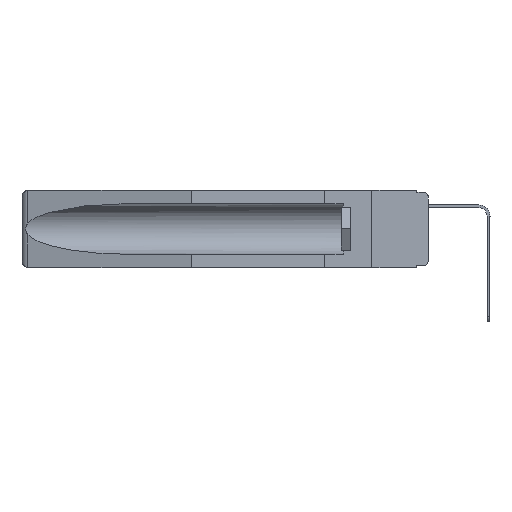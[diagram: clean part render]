
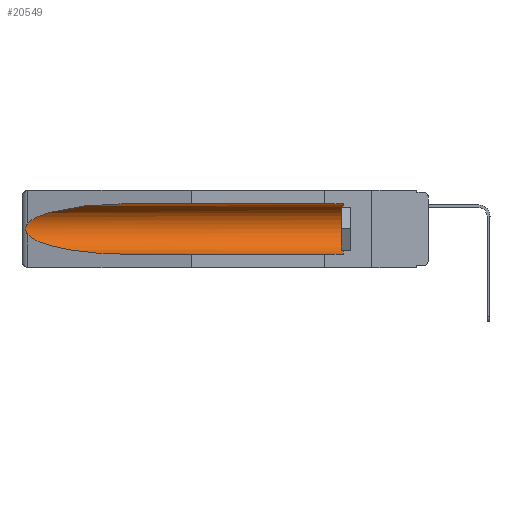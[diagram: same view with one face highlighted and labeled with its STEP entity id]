
A CAD part, left-side view. The second image highlights one B-rep face of the part: STEP entity #20549.
In plain terms, the highlighted cylindrical face has radius 2.857 mm (diameter 5.715 mm), a partial arc.
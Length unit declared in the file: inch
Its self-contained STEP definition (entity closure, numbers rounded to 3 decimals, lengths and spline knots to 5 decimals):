
#26 = VERTEX_POINT ( 'NONE', #24285 ) ;
#1350 = VERTEX_POINT ( 'NONE', #5769 ) ;
#1535 = CARTESIAN_POINT ( 'NONE',  ( 0.155, 1.07973, -0.284 ) ) ;
#2356 = ORIENTED_EDGE ( 'NONE', *, *, #2501, .T. ) ;
#2501 = EDGE_CURVE ( 'NONE', #20024, #16948, #13579, .T. ) ;
#2615 = CARTESIAN_POINT ( 'NONE',  ( 0.26654, 1.53092, -0.15636 ) ) ;
#2999 = FACE_OUTER_BOUND ( 'NONE', #20802, .T. ) ;
#3125 = CARTESIAN_POINT ( 'NONE',  ( 0.2675, 1.53308, -0.17534 ) ) ;
#3566 = ORIENTED_EDGE ( 'NONE', *, *, #14625, .T. ) ;
#3877 = CARTESIAN_POINT ( 'NONE',  ( 0.155, -0.30754, -0.284 ) ) ;
#4332 = CARTESIAN_POINT ( 'NONE',  ( 0.155, -0.30754, -0.1715 ) ) ;
#4775 = CARTESIAN_POINT ( 'NONE',  ( 0.26537, 1.52718, -0.19328 ) ) ;
#5769 = CARTESIAN_POINT ( 'NONE',  ( 0.155, 0.126, -0.284 ) ) ;
#6093 = ORIENTED_EDGE ( 'NONE', *, *, #7847, .F. ) ;
#6315 = CARTESIAN_POINT ( 'NONE',  ( 0.155, -0.30754, -0.059 ) ) ;
#6338 = DIRECTION ( 'NONE',  ( 0., 1., 0. ) ) ;
#6850 =( BOUNDED_CURVE ( )  B_SPLINE_CURVE ( 3, ( #9888, #23313, #19418, #12179 ),
 .UNSPECIFIED., .F., .F. ) 
 B_SPLINE_CURVE_WITH_KNOTS ( ( 4, 4 ),
 ( 4.71239, 6.08839 ),
 .UNSPECIFIED. ) 
 CURVE ( )  GEOMETRIC_REPRESENTATION_ITEM ( )  RATIONAL_B_SPLINE_CURVE ( ( 1., 0.848, 0.848, 1. ) ) 
 REPRESENTATION_ITEM ( '' )  );
#6964 = CARTESIAN_POINT ( 'NONE',  ( 0.26655, 1.53094, -0.18657 ) ) ;
#7096 = CARTESIAN_POINT ( 'NONE',  ( 0.21114, 1.30732, -0.284 ) ) ;
#7478 = CYLINDRICAL_SURFACE ( 'NONE', #15297, 0.1125 ) ;
#7492 = DIRECTION ( 'NONE',  ( 0., -1., 0. ) ) ;
#7847 = EDGE_CURVE ( 'NONE', #1350, #23881, #13868, .T. ) ;
#8426 = CARTESIAN_POINT ( 'NONE',  ( 0.26537, 1.52718, -0.14972 ) ) ;
#8512 = CARTESIAN_POINT ( 'NONE',  ( 0.2673, 1.5327, -0.16383 ) ) ;
#8907 = CARTESIAN_POINT ( 'NONE',  ( 0.155, 1.07973, -0.284 ) ) ;
#9697 = AXIS2_PLACEMENT_3D ( 'NONE', #18843, #7492, #20726 ) ;
#9840 = EDGE_CURVE ( 'NONE', #1350, #20024, #19397, .T. ) ;
#9888 = CARTESIAN_POINT ( 'NONE',  ( 0.155, 1.07973, -0.059 ) ) ;
#10599 = CARTESIAN_POINT ( 'NONE',  ( 0.2673, 1.53269, -0.17917 ) ) ;
#11161 = CARTESIAN_POINT ( 'NONE',  ( 0.26537, 1.52718, -0.14972 ) ) ;
#11179 = VECTOR ( 'NONE', #17166, 39.37008 ) ;
#12013 = EDGE_CURVE ( 'NONE', #16948, #20307, #6850, .T. ) ;
#12179 = CARTESIAN_POINT ( 'NONE',  ( 0.26537, 1.52718, -0.14972 ) ) ;
#12754 = CARTESIAN_POINT ( 'NONE',  ( 0.2675, 1.53308, -0.16763 ) ) ;
#13579 = LINE ( 'NONE', #6315, #23342 ) ;
#13856 =( BOUNDED_CURVE ( )  B_SPLINE_CURVE ( 3, ( #16546, #23916, #7096, #8907 ),
 .UNSPECIFIED., .F., .F. ) 
 B_SPLINE_CURVE_WITH_KNOTS ( ( 4, 4 ),
 ( 0.1948, 1.5708 ),
 .UNSPECIFIED. ) 
 CURVE ( )  GEOMETRIC_REPRESENTATION_ITEM ( )  RATIONAL_B_SPLINE_CURVE ( ( 1., 0.848, 0.848, 1. ) ) 
 REPRESENTATION_ITEM ( '' )  );
#13868 = LINE ( 'NONE', #3877, #11179 ) ;
#14042 = DIRECTION ( 'NONE',  ( 0., 1., 0. ) ) ;
#14605 = CARTESIAN_POINT ( 'NONE',  ( 0.26597, 1.5296, -0.19026 ) ) ;
#14625 = EDGE_CURVE ( 'NONE', #20307, #26, #16436, .T. ) ;
#15297 = AXIS2_PLACEMENT_3D ( 'NONE', #4332, #6338, #15637 ) ;
#15585 = ORIENTED_EDGE ( 'NONE', *, *, #9840, .T. ) ;
#15637 = DIRECTION ( 'NONE',  ( 0., 0., 1. ) ) ;
#15988 = CARTESIAN_POINT ( 'NONE',  ( 0.26597, 1.52961, -0.15275 ) ) ;
#16436 = B_SPLINE_CURVE_WITH_KNOTS ( 'NONE', 3,
 ( #8426, #15988, #2615, #8512, #12754, #3125, #10599, #6964, #14605, #4775 ),
 .UNSPECIFIED., .F., .F.,
 ( 4, 2, 2, 2, 4 ),
 ( 0., 0.00029, 0.00058, 0.00087, 0.00117 ),
 .UNSPECIFIED. ) ;
#16546 = CARTESIAN_POINT ( 'NONE',  ( 0.26537, 1.52718, -0.19328 ) ) ;
#16948 = VERTEX_POINT ( 'NONE', #17722 ) ;
#17166 = DIRECTION ( 'NONE',  ( 0., 1., 0. ) ) ;
#17722 = CARTESIAN_POINT ( 'NONE',  ( 0.155, 1.07973, -0.059 ) ) ;
#18843 = CARTESIAN_POINT ( 'NONE',  ( 0.155, 0.126, -0.1715 ) ) ;
#19282 = ORIENTED_EDGE ( 'NONE', *, *, #20787, .T. ) ;
#19397 = CIRCLE ( 'NONE', #9697, 0.1125 ) ;
#19418 = CARTESIAN_POINT ( 'NONE',  ( 0.25451, 1.48313, -0.09465 ) ) ;
#20024 = VERTEX_POINT ( 'NONE', #23691 ) ;
#20307 = VERTEX_POINT ( 'NONE', #11161 ) ;
#20549 = ADVANCED_FACE ( 'NONE', ( #2999 ), #7478, .F. ) ;
#20726 = DIRECTION ( 'NONE',  ( 0., 0., 1. ) ) ;
#20780 = ORIENTED_EDGE ( 'NONE', *, *, #12013, .T. ) ;
#20787 = EDGE_CURVE ( 'NONE', #26, #23881, #13856, .T. ) ;
#20802 = EDGE_LOOP ( 'NONE', ( #20780, #3566, #19282, #6093, #15585, #2356 ) ) ;
#23313 = CARTESIAN_POINT ( 'NONE',  ( 0.21114, 1.30732, -0.059 ) ) ;
#23342 = VECTOR ( 'NONE', #14042, 39.37008 ) ;
#23691 = CARTESIAN_POINT ( 'NONE',  ( 0.155, 0.126, -0.059 ) ) ;
#23881 = VERTEX_POINT ( 'NONE', #1535 ) ;
#23916 = CARTESIAN_POINT ( 'NONE',  ( 0.25451, 1.48313, -0.24835 ) ) ;
#24285 = CARTESIAN_POINT ( 'NONE',  ( 0.26537, 1.52718, -0.19328 ) ) ;
